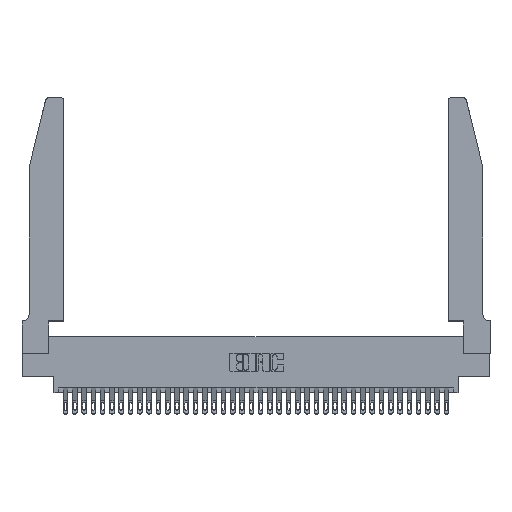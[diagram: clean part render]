
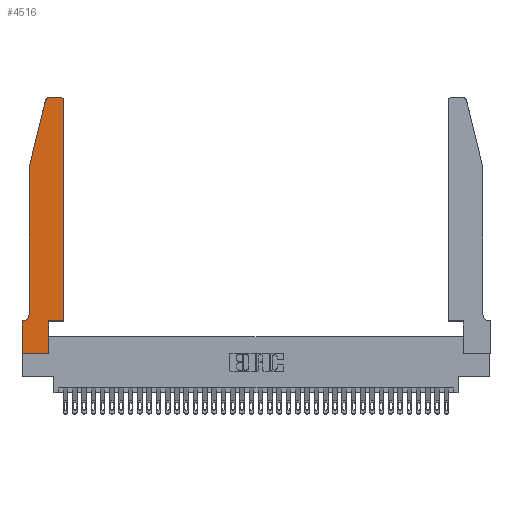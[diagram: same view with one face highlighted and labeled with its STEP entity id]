
A CAD part, top view. The second image highlights one B-rep face of the part: STEP entity #4516.
In plain terms, the highlighted planar face has unit normal (0, 0, 1).
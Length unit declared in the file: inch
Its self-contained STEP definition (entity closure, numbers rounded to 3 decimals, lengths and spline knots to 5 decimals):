
#288 = EDGE_CURVE ( 'NONE', #35145, #12171, #17660, .T. ) ;
#1676 = DIRECTION ( 'NONE',  ( 0., 0., 1. ) ) ;
#1694 = ORIENTED_EDGE ( 'NONE', *, *, #31466, .T. ) ;
#2180 = VERTEX_POINT ( 'NONE', #8050 ) ;
#2188 = CARTESIAN_POINT ( 'NONE',  ( 0., 0., 0.37 ) ) ;
#2213 = FACE_OUTER_BOUND ( 'NONE', #31888, .T. ) ;
#2279 = CARTESIAN_POINT ( 'NONE',  ( 0.2865, 0.35, 0.37 ) ) ;
#2716 = CARTESIAN_POINT ( 'NONE',  ( 0.4205, 2.72, 0.37 ) ) ;
#2843 = DIRECTION ( 'NONE',  ( 0., 1., 0. ) ) ;
#2982 = CARTESIAN_POINT ( 'NONE',  ( 0.4205, 2.75, 0.37 ) ) ;
#3514 = DIRECTION ( 'NONE',  ( 1., 0., 0. ) ) ;
#4146 = CARTESIAN_POINT ( 'NONE',  ( 0.2865, 0.35, 0.37 ) ) ;
#4516 = ADVANCED_FACE ( 'NONE', ( #2213 ), #35375, .T. ) ;
#4840 = VECTOR ( 'NONE', #28700, 39.37008 ) ;
#5390 = LINE ( 'NONE', #34475, #24684 ) ;
#5988 = LINE ( 'NONE', #24956, #21254 ) ;
#6478 = VERTEX_POINT ( 'NONE', #29170 ) ;
#7106 = CIRCLE ( 'NONE', #21226, 0.07 ) ;
#7348 = DIRECTION ( 'NONE',  ( 1., 0., 0. ) ) ;
#7653 = CARTESIAN_POINT ( 'NONE',  ( 0.0055, 0.42, 0.37 ) ) ;
#7724 = EDGE_CURVE ( 'NONE', #30022, #6478, #33294, .T. ) ;
#8050 = CARTESIAN_POINT ( 'NONE',  ( 0.25487, 2.72718, 0.37 ) ) ;
#8080 = CARTESIAN_POINT ( 'NONE',  ( 0.0055, 0.35, 0.37 ) ) ;
#8121 = CARTESIAN_POINT ( 'NONE',  ( 0.0755, 0.35, 0.37 ) ) ;
#8377 = EDGE_CURVE ( 'NONE', #11558, #30022, #5988, .T. ) ;
#8701 = CARTESIAN_POINT ( 'NONE',  ( 0.2605, 2.75, 0.37 ) ) ;
#9175 = VECTOR ( 'NONE', #35088, 39.37008 ) ;
#9548 = CIRCLE ( 'NONE', #28809, 0.03 ) ;
#10029 = EDGE_CURVE ( 'NONE', #23905, #2180, #9548, .T. ) ;
#10077 = EDGE_CURVE ( 'NONE', #21669, #28826, #5390, .T. ) ;
#10818 = CARTESIAN_POINT ( 'NONE',  ( 0.0755, 0.42, 0.37 ) ) ;
#11558 = VERTEX_POINT ( 'NONE', #25669 ) ;
#11730 = EDGE_CURVE ( 'NONE', #28826, #23520, #7106, .T. ) ;
#11803 = DIRECTION ( 'NONE',  ( 0., 0., 1. ) ) ;
#12171 = VERTEX_POINT ( 'NONE', #35957 ) ;
#12532 = ORIENTED_EDGE ( 'NONE', *, *, #22910, .T. ) ;
#12565 = CIRCLE ( 'NONE', #34280, 0.03 ) ;
#14202 = DIRECTION ( 'NONE',  ( 0., 0., 1. ) ) ;
#14296 = DIRECTION ( 'NONE',  ( 0., -1., 0. ) ) ;
#15155 = ORIENTED_EDGE ( 'NONE', *, *, #19043, .T. ) ;
#15374 = VECTOR ( 'NONE', #37106, 39.37008 ) ;
#15632 = CARTESIAN_POINT ( 'NONE',  ( 0.4505, 0.35, 0.37 ) ) ;
#15877 = DIRECTION ( 'NONE',  ( -1., 0., 0. ) ) ;
#16117 = CARTESIAN_POINT ( 'NONE',  ( 0.0755, 2., 0.37 ) ) ;
#16233 = DIRECTION ( 'NONE',  ( 0., -1., 0. ) ) ;
#16966 = DIRECTION ( 'NONE',  ( -0.239, -0.971, 0. ) ) ;
#16989 = ORIENTED_EDGE ( 'NONE', *, *, #288, .T. ) ;
#17660 = LINE ( 'NONE', #19726, #32363 ) ;
#18080 = ORIENTED_EDGE ( 'NONE', *, *, #10077, .T. ) ;
#18938 = CARTESIAN_POINT ( 'NONE',  ( 0., 0., 0.37 ) ) ;
#19043 = EDGE_CURVE ( 'NONE', #2180, #21669, #34486, .T. ) ;
#19297 = ORIENTED_EDGE ( 'NONE', *, *, #33208, .T. ) ;
#19434 = VECTOR ( 'NONE', #25107, 39.37008 ) ;
#19726 = CARTESIAN_POINT ( 'NONE',  ( 0.4505, 0.35, 0.37 ) ) ;
#19864 = DIRECTION ( 'NONE',  ( 1., 0., 0. ) ) ;
#21226 = AXIS2_PLACEMENT_3D ( 'NONE', #7653, #28230, #15877 ) ;
#21254 = VECTOR ( 'NONE', #16233, 39.37008 ) ;
#21669 = VERTEX_POINT ( 'NONE', #16117 ) ;
#22066 = ORIENTED_EDGE ( 'NONE', *, *, #24418, .T. ) ;
#22910 = EDGE_CURVE ( 'NONE', #6478, #28143, #36505, .T. ) ;
#23300 = LINE ( 'NONE', #8121, #4840 ) ;
#23520 = VERTEX_POINT ( 'NONE', #8080 ) ;
#23905 = VERTEX_POINT ( 'NONE', #35985 ) ;
#24418 = EDGE_CURVE ( 'NONE', #28143, #35145, #35970, .T. ) ;
#24684 = VECTOR ( 'NONE', #14296, 39.37008 ) ;
#24956 = CARTESIAN_POINT ( 'NONE',  ( 0., 0., 0.37 ) ) ;
#25107 = DIRECTION ( 'NONE',  ( 0., 1., 0. ) ) ;
#25669 = CARTESIAN_POINT ( 'NONE',  ( 0., 0.35, 0.37 ) ) ;
#26548 = AXIS2_PLACEMENT_3D ( 'NONE', #36391, #11803, #3514 ) ;
#27181 = CARTESIAN_POINT ( 'NONE',  ( 0.4505, 0.35, 0.37 ) ) ;
#28143 = VERTEX_POINT ( 'NONE', #2279 ) ;
#28230 = DIRECTION ( 'NONE',  ( 0., 0., -1. ) ) ;
#28309 = VERTEX_POINT ( 'NONE', #2982 ) ;
#28515 = LINE ( 'NONE', #8701, #9175 ) ;
#28700 = DIRECTION ( 'NONE',  ( -1., 0., 0. ) ) ;
#28809 = AXIS2_PLACEMENT_3D ( 'NONE', #32354, #1676, #7348 ) ;
#28826 = VERTEX_POINT ( 'NONE', #10818 ) ;
#29170 = CARTESIAN_POINT ( 'NONE',  ( 0.2865, 0., 0.37 ) ) ;
#29933 = VECTOR ( 'NONE', #19864, 39.37008 ) ;
#30022 = VERTEX_POINT ( 'NONE', #2188 ) ;
#30455 = ORIENTED_EDGE ( 'NONE', *, *, #36800, .T. ) ;
#30573 = ORIENTED_EDGE ( 'NONE', *, *, #8377, .T. ) ;
#31466 = EDGE_CURVE ( 'NONE', #23520, #11558, #23300, .T. ) ;
#31888 = EDGE_LOOP ( 'NONE', ( #30455, #34515, #15155, #18080, #33977, #1694, #30573, #35169, #12532, #22066, #16989, #19297 ) ) ;
#32354 = CARTESIAN_POINT ( 'NONE',  ( 0.284, 2.72, 0.37 ) ) ;
#32363 = VECTOR ( 'NONE', #2843, 39.37008 ) ;
#33208 = EDGE_CURVE ( 'NONE', #12171, #28309, #12565, .T. ) ;
#33294 = LINE ( 'NONE', #18938, #15374 ) ;
#33977 = ORIENTED_EDGE ( 'NONE', *, *, #11730, .T. ) ;
#34088 = CARTESIAN_POINT ( 'NONE',  ( 0.0755, 2., 0.37 ) ) ;
#34280 = AXIS2_PLACEMENT_3D ( 'NONE', #2716, #14202, #37902 ) ;
#34475 = CARTESIAN_POINT ( 'NONE',  ( 0.0755, 2., 0.37 ) ) ;
#34486 = LINE ( 'NONE', #34088, #36776 ) ;
#34515 = ORIENTED_EDGE ( 'NONE', *, *, #10029, .T. ) ;
#35088 = DIRECTION ( 'NONE',  ( -1., 0., 0. ) ) ;
#35145 = VERTEX_POINT ( 'NONE', #27181 ) ;
#35169 = ORIENTED_EDGE ( 'NONE', *, *, #7724, .T. ) ;
#35375 = PLANE ( 'NONE',  #26548 ) ;
#35957 = CARTESIAN_POINT ( 'NONE',  ( 0.4505, 2.72, 0.37 ) ) ;
#35970 = LINE ( 'NONE', #15632, #29933 ) ;
#35985 = CARTESIAN_POINT ( 'NONE',  ( 0.284, 2.75, 0.37 ) ) ;
#36391 = CARTESIAN_POINT ( 'NONE',  ( 0., 0.35, 0.37 ) ) ;
#36505 = LINE ( 'NONE', #4146, #19434 ) ;
#36776 = VECTOR ( 'NONE', #16966, 39.37008 ) ;
#36800 = EDGE_CURVE ( 'NONE', #28309, #23905, #28515, .T. ) ;
#37106 = DIRECTION ( 'NONE',  ( 1., 0., 0. ) ) ;
#37902 = DIRECTION ( 'NONE',  ( 1., 0., 0. ) ) ;
